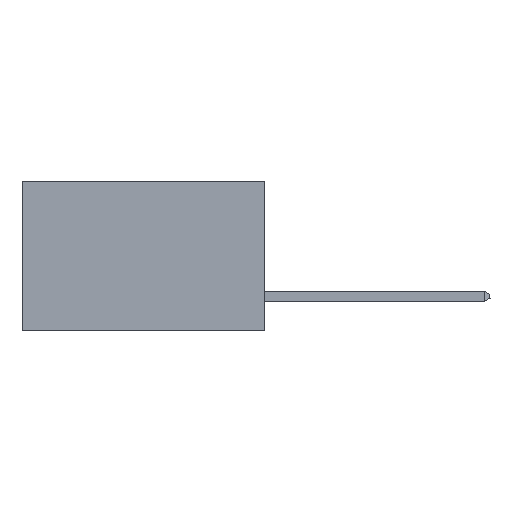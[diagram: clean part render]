
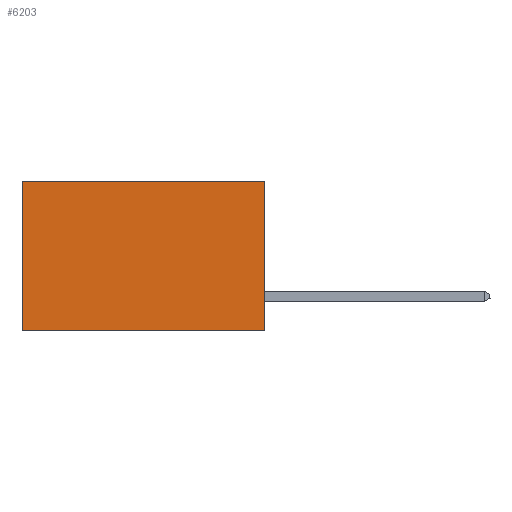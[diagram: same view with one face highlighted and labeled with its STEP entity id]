
A CAD part, left-side view. The second image highlights one B-rep face of the part: STEP entity #6203.
In plain terms, the highlighted planar face has unit normal (-1, 0, 0).
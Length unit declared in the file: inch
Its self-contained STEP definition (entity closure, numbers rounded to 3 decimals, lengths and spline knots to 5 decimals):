
#121 = DIRECTION ( 'NONE',  ( 1., 0., 0. ) ) ;
#297 = DIRECTION ( 'NONE',  ( 0., 1., 0. ) ) ;
#384 = ORIENTED_EDGE ( 'NONE', *, *, #963, .T. ) ;
#524 = ORIENTED_EDGE ( 'NONE', *, *, #6163, .T. ) ;
#963 = EDGE_CURVE ( 'NONE', #8517, #4944, #5303, .T. ) ;
#1249 = FACE_OUTER_BOUND ( 'NONE', #4566, .T. ) ;
#1718 = LINE ( 'NONE', #7448, #2439 ) ;
#2238 = VECTOR ( 'NONE', #297, 39.37008 ) ;
#2439 = VECTOR ( 'NONE', #7432, 39.37008 ) ;
#2450 = VERTEX_POINT ( 'NONE', #4949 ) ;
#3135 = EDGE_CURVE ( 'NONE', #2450, #4944, #6520, .T. ) ;
#3217 = CARTESIAN_POINT ( 'NONE',  ( 0.298, 0.6, 0. ) ) ;
#3227 = EDGE_CURVE ( 'NONE', #3719, #2450, #8501, .T. ) ;
#3293 = VECTOR ( 'NONE', #3788, 39.37008 ) ;
#3719 = VERTEX_POINT ( 'NONE', #7819 ) ;
#3788 = DIRECTION ( 'NONE',  ( 0., 0., -1. ) ) ;
#4045 = CARTESIAN_POINT ( 'NONE',  ( 0.298, 0., 0. ) ) ;
#4566 = EDGE_LOOP ( 'NONE', ( #384, #5057, #4692, #524 ) ) ;
#4692 = ORIENTED_EDGE ( 'NONE', *, *, #3227, .F. ) ;
#4944 = VERTEX_POINT ( 'NONE', #5723 ) ;
#4949 = CARTESIAN_POINT ( 'NONE',  ( 0.298, 0., -0.37 ) ) ;
#5057 = ORIENTED_EDGE ( 'NONE', *, *, #3135, .F. ) ;
#5167 = VECTOR ( 'NONE', #5756, 39.37008 ) ;
#5303 = LINE ( 'NONE', #3217, #3293 ) ;
#5428 = CARTESIAN_POINT ( 'NONE',  ( 0.298, 0., 0. ) ) ;
#5486 = PLANE ( 'NONE',  #7972 ) ;
#5723 = CARTESIAN_POINT ( 'NONE',  ( 0.298, 0.6, -0.37 ) ) ;
#5756 = DIRECTION ( 'NONE',  ( 0., 0., -1. ) ) ;
#6163 = EDGE_CURVE ( 'NONE', #3719, #8517, #1718, .T. ) ;
#6203 = ADVANCED_FACE ( 'NONE', ( #1249 ), #5486, .F. ) ;
#6246 = DIRECTION ( 'NONE',  ( 0., 0., -1. ) ) ;
#6520 = LINE ( 'NONE', #6863, #2238 ) ;
#6863 = CARTESIAN_POINT ( 'NONE',  ( 0.298, 0., -0.37 ) ) ;
#7432 = DIRECTION ( 'NONE',  ( 0., 1., 0. ) ) ;
#7448 = CARTESIAN_POINT ( 'NONE',  ( 0.298, 0., 0. ) ) ;
#7819 = CARTESIAN_POINT ( 'NONE',  ( 0.298, 0., 0. ) ) ;
#7972 = AXIS2_PLACEMENT_3D ( 'NONE', #4045, #121, #6246 ) ;
#8103 = CARTESIAN_POINT ( 'NONE',  ( 0.298, 0.6, 0. ) ) ;
#8501 = LINE ( 'NONE', #5428, #5167 ) ;
#8517 = VERTEX_POINT ( 'NONE', #8103 ) ;
